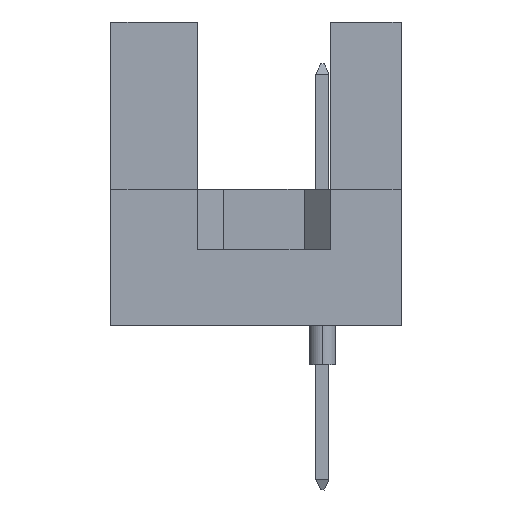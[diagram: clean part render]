
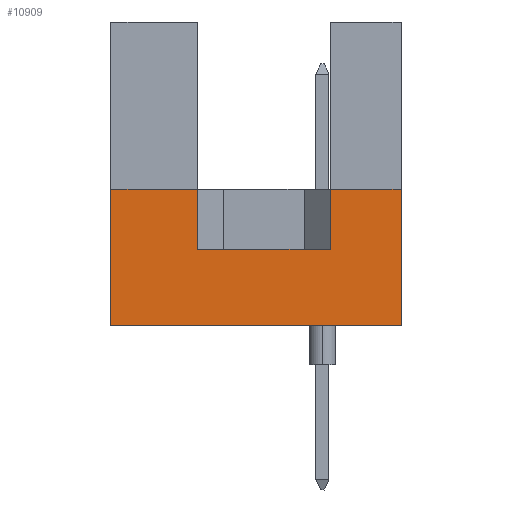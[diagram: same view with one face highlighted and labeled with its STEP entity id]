
A CAD part, left-side view. The second image highlights one B-rep face of the part: STEP entity #10909.
In plain terms, the highlighted planar face has unit normal (-1, 0, 0).
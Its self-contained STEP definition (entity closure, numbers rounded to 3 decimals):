
#2 = DIRECTION ( 'NONE',  ( 0., 0., -1. ) ) ;
#596 = CARTESIAN_POINT ( 'NONE',  ( -47.5, 11.1, 5.2 ) ) ;
#631 = EDGE_CURVE ( 'NONE', #13992, #12899, #6845, .T. ) ;
#745 = DIRECTION ( 'NONE',  ( 0., 0., 1. ) ) ;
#770 = VERTEX_POINT ( 'NONE', #6037 ) ;
#787 = CARTESIAN_POINT ( 'NONE',  ( -47.5, 2.71, 5.2 ) ) ;
#842 = DIRECTION ( 'NONE',  ( 0., -1., 0. ) ) ;
#866 = DIRECTION ( 'NONE',  ( 0., 0., 1. ) ) ;
#937 = LINE ( 'NONE', #8326, #3146 ) ;
#1078 = ORIENTED_EDGE ( 'NONE', *, *, #631, .F. ) ;
#1181 = CARTESIAN_POINT ( 'NONE',  ( -47.5, 11.1, 0. ) ) ;
#1614 = EDGE_CURVE ( 'NONE', #4517, #10522, #3700, .T. ) ;
#2057 = ORIENTED_EDGE ( 'NONE', *, *, #14238, .T. ) ;
#2126 = ORIENTED_EDGE ( 'NONE', *, *, #12961, .T. ) ;
#2774 = VERTEX_POINT ( 'NONE', #13213 ) ;
#3146 = VECTOR ( 'NONE', #4673, 1000. ) ;
#3623 = LINE ( 'NONE', #12941, #10519 ) ;
#3700 = LINE ( 'NONE', #16068, #15423 ) ;
#4354 = VERTEX_POINT ( 'NONE', #5487 ) ;
#4517 = VERTEX_POINT ( 'NONE', #1181 ) ;
#4673 = DIRECTION ( 'NONE',  ( 0., 0., 1. ) ) ;
#4864 = ORIENTED_EDGE ( 'NONE', *, *, #10285, .F. ) ;
#4967 = VECTOR ( 'NONE', #745, 1000. ) ;
#5487 = CARTESIAN_POINT ( 'NONE',  ( -47.5, 0., 5.2 ) ) ;
#5777 = LINE ( 'NONE', #13109, #7513 ) ;
#6037 = CARTESIAN_POINT ( 'NONE',  ( -47.5, 7.79, 5.2 ) ) ;
#6044 = CARTESIAN_POINT ( 'NONE',  ( -47.5, 7.79, 2.9 ) ) ;
#6319 = DIRECTION ( 'NONE',  ( 1., 0., 0. ) ) ;
#6838 = LINE ( 'NONE', #596, #11959 ) ;
#6845 = LINE ( 'NONE', #13189, #7636 ) ;
#6918 = CARTESIAN_POINT ( 'NONE',  ( -47.5, 7.79, 2.9 ) ) ;
#7513 = VECTOR ( 'NONE', #10496, 1000. ) ;
#7533 = PLANE ( 'NONE',  #12705 ) ;
#7636 = VECTOR ( 'NONE', #842, 1000. ) ;
#7725 = DIRECTION ( 'NONE',  ( 0., -1., 0. ) ) ;
#8137 = LINE ( 'NONE', #6918, #4967 ) ;
#8326 = CARTESIAN_POINT ( 'NONE',  ( -47.5, 0., 0. ) ) ;
#8917 = LINE ( 'NONE', #15420, #11162 ) ;
#9178 = EDGE_CURVE ( 'NONE', #9356, #4354, #8917, .T. ) ;
#9356 = VERTEX_POINT ( 'NONE', #787 ) ;
#9846 = ORIENTED_EDGE ( 'NONE', *, *, #14152, .T. ) ;
#9996 = CARTESIAN_POINT ( 'NONE',  ( -47.5, 11.1, 5.2 ) ) ;
#10115 = DIRECTION ( 'NONE',  ( 0., 0., 1. ) ) ;
#10285 = EDGE_CURVE ( 'NONE', #10522, #770, #6838, .T. ) ;
#10496 = DIRECTION ( 'NONE',  ( 0., -1., 0. ) ) ;
#10519 = VECTOR ( 'NONE', #10115, 1000. ) ;
#10522 = VERTEX_POINT ( 'NONE', #9996 ) ;
#10909 = ADVANCED_FACE ( 'NONE', ( #11043 ), #7533, .F. ) ;
#10987 = ORIENTED_EDGE ( 'NONE', *, *, #9178, .F. ) ;
#11043 = FACE_OUTER_BOUND ( 'NONE', #11666, .T. ) ;
#11162 = VECTOR ( 'NONE', #14202, 1000. ) ;
#11666 = EDGE_LOOP ( 'NONE', ( #1078, #2057, #4864, #12294, #9846, #2126, #10987, #14237 ) ) ;
#11959 = VECTOR ( 'NONE', #7725, 1000. ) ;
#12294 = ORIENTED_EDGE ( 'NONE', *, *, #1614, .F. ) ;
#12705 = AXIS2_PLACEMENT_3D ( 'NONE', #13568, #6319, #2 ) ;
#12899 = VERTEX_POINT ( 'NONE', #15724 ) ;
#12941 = CARTESIAN_POINT ( 'NONE',  ( -47.5, 2.71, 2.9 ) ) ;
#12961 = EDGE_CURVE ( 'NONE', #2774, #4354, #937, .T. ) ;
#13109 = CARTESIAN_POINT ( 'NONE',  ( -47.5, 11.1, 0. ) ) ;
#13189 = CARTESIAN_POINT ( 'NONE',  ( -47.5, 7.79, 2.9 ) ) ;
#13213 = CARTESIAN_POINT ( 'NONE',  ( -47.5, 0., 0. ) ) ;
#13568 = CARTESIAN_POINT ( 'NONE',  ( -47.5, 11.1, 0. ) ) ;
#13992 = VERTEX_POINT ( 'NONE', #6044 ) ;
#14152 = EDGE_CURVE ( 'NONE', #4517, #2774, #5777, .T. ) ;
#14202 = DIRECTION ( 'NONE',  ( 0., -1., 0. ) ) ;
#14237 = ORIENTED_EDGE ( 'NONE', *, *, #15240, .F. ) ;
#14238 = EDGE_CURVE ( 'NONE', #13992, #770, #8137, .T. ) ;
#15240 = EDGE_CURVE ( 'NONE', #12899, #9356, #3623, .T. ) ;
#15420 = CARTESIAN_POINT ( 'NONE',  ( -47.5, 11.1, 5.2 ) ) ;
#15423 = VECTOR ( 'NONE', #866, 1000. ) ;
#15724 = CARTESIAN_POINT ( 'NONE',  ( -47.5, 2.71, 2.9 ) ) ;
#16068 = CARTESIAN_POINT ( 'NONE',  ( -47.5, 11.1, 0. ) ) ;
